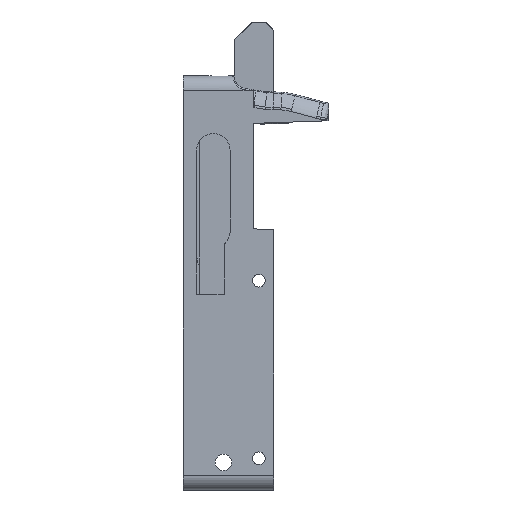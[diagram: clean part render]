
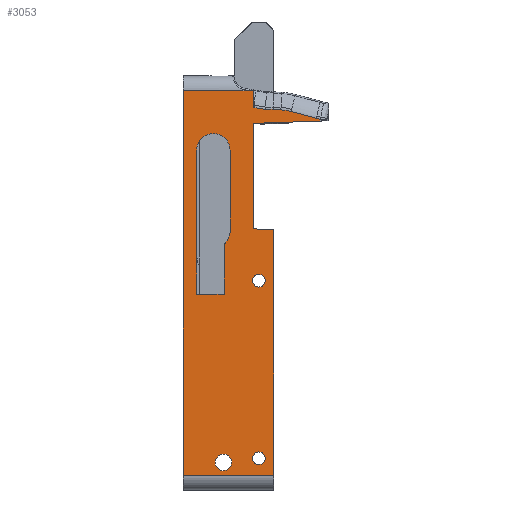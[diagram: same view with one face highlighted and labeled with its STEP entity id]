
A CAD part, left-side view. The second image highlights one B-rep face of the part: STEP entity #3053.
In plain terms, the highlighted planar face has unit normal (-1, 0, 0).
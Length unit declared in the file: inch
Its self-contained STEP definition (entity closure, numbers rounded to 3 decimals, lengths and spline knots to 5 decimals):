
#41=FACE_BOUND('',#860,.T.);
#42=FACE_BOUND('',#861,.T.);
#43=FACE_BOUND('',#862,.T.);
#44=FACE_BOUND('',#863,.T.);
#69=PLANE('',#3259);
#131=LINE('',#4481,#373);
#135=LINE('',#4535,#377);
#158=LINE('',#4780,#400);
#159=LINE('',#4782,#401);
#160=LINE('',#4784,#402);
#161=LINE('',#4786,#403);
#162=LINE('',#4788,#404);
#163=LINE('',#4790,#405);
#164=LINE('',#4792,#406);
#165=LINE('',#4794,#407);
#166=LINE('',#4796,#408);
#167=LINE('',#4798,#409);
#168=LINE('',#4805,#410);
#169=LINE('',#4807,#411);
#170=LINE('',#4809,#412);
#171=LINE('',#4810,#413);
#172=LINE('',#4815,#414);
#173=LINE('',#4817,#415);
#174=LINE('',#4819,#416);
#175=LINE('',#4823,#417);
#373=VECTOR('',#3537,0.02);
#377=VECTOR('',#3545,0.3937);
#400=VECTOR('',#3610,0.3937);
#401=VECTOR('',#3611,0.3937);
#402=VECTOR('',#3612,0.3937);
#403=VECTOR('',#3613,0.3937);
#404=VECTOR('',#3614,0.3937);
#405=VECTOR('',#3615,0.3937);
#406=VECTOR('',#3616,0.3937);
#407=VECTOR('',#3617,0.3937);
#408=VECTOR('',#3618,0.3937);
#409=VECTOR('',#3619,0.3937);
#410=VECTOR('',#3620,0.3937);
#411=VECTOR('',#3621,0.3937);
#412=VECTOR('',#3622,0.3937);
#413=VECTOR('',#3623,0.3937);
#414=VECTOR('',#3626,0.3937);
#415=VECTOR('',#3627,0.3937);
#416=VECTOR('',#3628,0.3937);
#417=VECTOR('',#3631,0.3937);
#686=FACE_OUTER_BOUND('',#859,.T.);
#859=EDGE_LOOP('',(#2141,#2142,#2143,#2144,#2145,#2146,#2147,#2148,#2149,
#2150,#2151,#2152,#2153,#2154,#2155,#2156,#2157));
#860=EDGE_LOOP('',(#2158,#2159,#2160,#2161,#2162,#2163,#2164));
#861=EDGE_LOOP('',(#2165));
#862=EDGE_LOOP('',(#2166));
#863=EDGE_LOOP('',(#2167));
#1047=CIRCLE('',#3260,0.1);
#1048=CIRCLE('',#3261,0.25);
#1049=CIRCLE('',#3262,0.25);
#1050=CIRCLE('',#3263,0.125);
#1051=CIRCLE('',#3264,0.094);
#1052=CIRCLE('',#3265,0.094);
#1212=B_SPLINE_CURVE_WITH_KNOTS('',3,(#4800,#4801,#4802,#4803),
 .UNSPECIFIED.,.F.,.F.,(4,4),(-0.39206,0.00034),
 .UNSPECIFIED.);
#1276=VERTEX_POINT('',#4382);
#1280=VERTEX_POINT('',#4477);
#1284=VERTEX_POINT('',#4534);
#1322=VERTEX_POINT('',#4779);
#1323=VERTEX_POINT('',#4781);
#1324=VERTEX_POINT('',#4783);
#1325=VERTEX_POINT('',#4785);
#1326=VERTEX_POINT('',#4787);
#1327=VERTEX_POINT('',#4789);
#1328=VERTEX_POINT('',#4791);
#1329=VERTEX_POINT('',#4793);
#1330=VERTEX_POINT('',#4795);
#1331=VERTEX_POINT('',#4797);
#1332=VERTEX_POINT('',#4799);
#1333=VERTEX_POINT('',#4804);
#1334=VERTEX_POINT('',#4806);
#1335=VERTEX_POINT('',#4808);
#1336=VERTEX_POINT('',#4811);
#1337=VERTEX_POINT('',#4812);
#1338=VERTEX_POINT('',#4814);
#1339=VERTEX_POINT('',#4816);
#1340=VERTEX_POINT('',#4818);
#1341=VERTEX_POINT('',#4820);
#1342=VERTEX_POINT('',#4822);
#1343=VERTEX_POINT('',#4825);
#1344=VERTEX_POINT('',#4827);
#1345=VERTEX_POINT('',#4829);
#1596=EDGE_CURVE('',#1276,#1280,#131,.T.);
#1601=EDGE_CURVE('',#1284,#1280,#135,.T.);
#1646=EDGE_CURVE('',#1276,#1322,#158,.T.);
#1647=EDGE_CURVE('',#1323,#1322,#159,.T.);
#1648=EDGE_CURVE('',#1324,#1323,#160,.T.);
#1649=EDGE_CURVE('',#1324,#1325,#161,.T.);
#1650=EDGE_CURVE('',#1325,#1326,#162,.T.);
#1651=EDGE_CURVE('',#1326,#1327,#163,.T.);
#1652=EDGE_CURVE('',#1327,#1328,#164,.T.);
#1653=EDGE_CURVE('',#1329,#1328,#165,.T.);
#1654=EDGE_CURVE('',#1330,#1329,#166,.T.);
#1655=EDGE_CURVE('',#1331,#1330,#167,.T.);
#1656=EDGE_CURVE('',#1332,#1331,#1212,.T.);
#1657=EDGE_CURVE('',#1333,#1332,#168,.T.);
#1658=EDGE_CURVE('',#1334,#1333,#169,.T.);
#1659=EDGE_CURVE('',#1335,#1334,#170,.T.);
#1660=EDGE_CURVE('',#1335,#1284,#171,.T.);
#1661=EDGE_CURVE('',#1336,#1337,#1047,.T.);
#1662=EDGE_CURVE('',#1336,#1338,#172,.T.);
#1663=EDGE_CURVE('',#1338,#1339,#173,.T.);
#1664=EDGE_CURVE('',#1339,#1340,#174,.T.);
#1665=EDGE_CURVE('',#1340,#1341,#1048,.T.);
#1666=EDGE_CURVE('',#1341,#1342,#175,.T.);
#1667=EDGE_CURVE('',#1342,#1337,#1049,.T.);
#1668=EDGE_CURVE('',#1343,#1343,#1050,.T.);
#1669=EDGE_CURVE('',#1344,#1344,#1051,.T.);
#1670=EDGE_CURVE('',#1345,#1345,#1052,.T.);
#2141=ORIENTED_EDGE('',*,*,#1596,.F.);
#2142=ORIENTED_EDGE('',*,*,#1646,.T.);
#2143=ORIENTED_EDGE('',*,*,#1647,.F.);
#2144=ORIENTED_EDGE('',*,*,#1648,.F.);
#2145=ORIENTED_EDGE('',*,*,#1649,.T.);
#2146=ORIENTED_EDGE('',*,*,#1650,.T.);
#2147=ORIENTED_EDGE('',*,*,#1651,.T.);
#2148=ORIENTED_EDGE('',*,*,#1652,.T.);
#2149=ORIENTED_EDGE('',*,*,#1653,.F.);
#2150=ORIENTED_EDGE('',*,*,#1654,.F.);
#2151=ORIENTED_EDGE('',*,*,#1655,.F.);
#2152=ORIENTED_EDGE('',*,*,#1656,.F.);
#2153=ORIENTED_EDGE('',*,*,#1657,.F.);
#2154=ORIENTED_EDGE('',*,*,#1658,.F.);
#2155=ORIENTED_EDGE('',*,*,#1659,.F.);
#2156=ORIENTED_EDGE('',*,*,#1660,.T.);
#2157=ORIENTED_EDGE('',*,*,#1601,.T.);
#2158=ORIENTED_EDGE('',*,*,#1661,.F.);
#2159=ORIENTED_EDGE('',*,*,#1662,.T.);
#2160=ORIENTED_EDGE('',*,*,#1663,.T.);
#2161=ORIENTED_EDGE('',*,*,#1664,.T.);
#2162=ORIENTED_EDGE('',*,*,#1665,.T.);
#2163=ORIENTED_EDGE('',*,*,#1666,.T.);
#2164=ORIENTED_EDGE('',*,*,#1667,.T.);
#2165=ORIENTED_EDGE('',*,*,#1668,.T.);
#2166=ORIENTED_EDGE('',*,*,#1669,.T.);
#2167=ORIENTED_EDGE('',*,*,#1670,.T.);
#3053=ADVANCED_FACE('',(#686,#41,#42,#43,#44),#69,.T.);
#3259=AXIS2_PLACEMENT_3D('',#4778,#3608,#3609);
#3260=AXIS2_PLACEMENT_3D('',#4813,#3624,#3625);
#3261=AXIS2_PLACEMENT_3D('',#4821,#3629,#3630);
#3262=AXIS2_PLACEMENT_3D('',#4824,#3632,#3633);
#3263=AXIS2_PLACEMENT_3D('',#4826,#3634,#3635);
#3264=AXIS2_PLACEMENT_3D('',#4828,#3636,#3637);
#3265=AXIS2_PLACEMENT_3D('',#4830,#3638,#3639);
#3537=DIRECTION('',(0.,-0.988,-0.151));
#3545=DIRECTION('',(0.,0.,1.));
#3608=DIRECTION('center_axis',(-1.,0.,0.));
#3609=DIRECTION('ref_axis',(0.,0.,1.));
#3610=DIRECTION('',(0.,1.,0.));
#3611=DIRECTION('',(0.,0.,1.));
#3612=DIRECTION('',(0.,1.,0.));
#3613=DIRECTION('',(0.,0.,1.));
#3614=DIRECTION('',(0.,0.999,0.035));
#3615=DIRECTION('',(0.,0.,1.));
#3616=DIRECTION('',(0.,-0.999,0.035));
#3617=DIRECTION('',(0.,0.,-1.));
#3618=DIRECTION('',(0.,-0.972,-0.233));
#3619=DIRECTION('',(0.,-0.966,-0.259));
#3620=DIRECTION('',(0.,-0.999,-0.052));
#3621=DIRECTION('',(0.,-1.,0.));
#3622=DIRECTION('',(0.,-0.988,-0.151));
#3623=DIRECTION('',(0.,0.995,0.099));
#3624=DIRECTION('center_axis',(1.,0.,0.));
#3625=DIRECTION('ref_axis',(0.,0.934,0.359));
#3626=DIRECTION('',(0.,0.,-1.));
#3627=DIRECTION('',(0.,1.,0.));
#3628=DIRECTION('',(0.,0.,1.));
#3629=DIRECTION('center_axis',(1.,0.,0.));
#3630=DIRECTION('ref_axis',(0.,1.,0.));
#3631=DIRECTION('',(0.,0.,-1.));
#3632=DIRECTION('center_axis',(1.,0.,0.));
#3633=DIRECTION('ref_axis',(0.,-1.,0.));
#3634=DIRECTION('center_axis',(1.,0.,0.));
#3635=DIRECTION('ref_axis',(0.,0.,-1.));
#3636=DIRECTION('center_axis',(1.,0.,0.));
#3637=DIRECTION('ref_axis',(0.,0.,-1.));
#3638=DIRECTION('center_axis',(1.,0.,0.));
#3639=DIRECTION('ref_axis',(0.,0.,-1.));
#4382=CARTESIAN_POINT('',(0.,1.21678,-1.025));
#4477=CARTESIAN_POINT('',(0.,1.1565,-1.03423));
#4481=CARTESIAN_POINT('',(0.,-0.86612,-1.34396));
#4534=CARTESIAN_POINT('',(0.,1.1565,-1.28015));
#4535=CARTESIAN_POINT('',(0.,1.1565,-4.07406));
#4778=CARTESIAN_POINT('Origin',(0.,0.,-7.));
#4779=CARTESIAN_POINT('',(0.,2.2,-1.025));
#4780=CARTESIAN_POINT('',(0.,1.42866,-1.025));
#4781=CARTESIAN_POINT('',(0.,2.2,-6.78));
#4782=CARTESIAN_POINT('',(0.,2.2,-7.));
#4783=CARTESIAN_POINT('',(0.,0.85,-6.78));
#4784=CARTESIAN_POINT('',(0.,0.,-6.78));
#4785=CARTESIAN_POINT('',(0.,0.85,-3.10499));
#4786=CARTESIAN_POINT('',(0.,0.85,-5.0625));
#4787=CARTESIAN_POINT('',(0.,1.1565,-3.09428));
#4788=CARTESIAN_POINT('',(0.,0.35724,-3.1222));
#4789=CARTESIAN_POINT('',(0.,1.1565,-1.51637));
#4790=CARTESIAN_POINT('',(0.,1.1565,-3.15463));
#4791=CARTESIAN_POINT('',(0.,0.14881,-1.48118));
#4792=CARTESIAN_POINT('',(0.,0.68375,-1.49986));
#4793=CARTESIAN_POINT('',(0.,0.14881,-1.45494));
#4794=CARTESIAN_POINT('',(0.,0.14881,-7.));
#4795=CARTESIAN_POINT('',(0.,0.21053,-1.44012));
#4796=CARTESIAN_POINT('',(0.,0.21008,-1.44023));
#4797=CARTESIAN_POINT('',(0.,0.58866,-1.3388));
#4798=CARTESIAN_POINT('',(0.,0.58438,-1.33995));
#4799=CARTESIAN_POINT('',(0.,0.74077,-1.31348));
#4800=CARTESIAN_POINT('Ctrl Pts',(0.,0.74077,
-1.31348));
#4801=CARTESIAN_POINT('Ctrl Pts',(0.,0.68937,
-1.31658));
#4802=CARTESIAN_POINT('Ctrl Pts',(0.,0.63829,
-1.32508));
#4803=CARTESIAN_POINT('Ctrl Pts',(0.,0.58866,
-1.3388));
#4804=CARTESIAN_POINT('',(0.,0.85687,-1.30739));
#4805=CARTESIAN_POINT('',(0.,0.8535,-1.30757));
#4806=CARTESIAN_POINT('',(0.,0.97402,-1.30739));
#4807=CARTESIAN_POINT('',(0.,0.98384,-1.30739));
#4808=CARTESIAN_POINT('',(0.,1.14343,-1.28145));
#4809=CARTESIAN_POINT('',(0.,1.13675,-1.28248));
#4810=CARTESIAN_POINT('',(0.,1.14343,-1.28145));
#4811=CARTESIAN_POINT('',(0.,1.59,-3.36221));
#4812=CARTESIAN_POINT('',(0.,1.56429,-3.29527));
#4813=CARTESIAN_POINT('Origin',(0.,1.49,-3.36221));
#4814=CARTESIAN_POINT('',(0.,1.59,-4.07));
#4815=CARTESIAN_POINT('',(0.,1.59,-5.535));
#4816=CARTESIAN_POINT('',(0.,2.,-4.07));
#4817=CARTESIAN_POINT('',(0.,1.,-4.07));
#4818=CARTESIAN_POINT('',(0.,2.,-1.92));
#4819=CARTESIAN_POINT('',(0.,2.,-4.46));
#4820=CARTESIAN_POINT('',(0.,1.5,-1.92));
#4821=CARTESIAN_POINT('Origin',(0.,1.75,-1.92));
#4822=CARTESIAN_POINT('',(0.,1.5,-3.12791));
#4823=CARTESIAN_POINT('',(0.,1.5,-5.06395));
#4824=CARTESIAN_POINT('Origin',(0.,1.75,-3.12791));
#4825=CARTESIAN_POINT('',(0.,1.6,-6.462));
#4826=CARTESIAN_POINT('Origin',(0.,1.6,-6.587));
#4827=CARTESIAN_POINT('',(0.,1.07,-6.431));
#4828=CARTESIAN_POINT('Origin',(0.,1.07,-6.525));
#4829=CARTESIAN_POINT('',(0.,1.07,-3.776));
#4830=CARTESIAN_POINT('Origin',(0.,1.07,-3.87));
